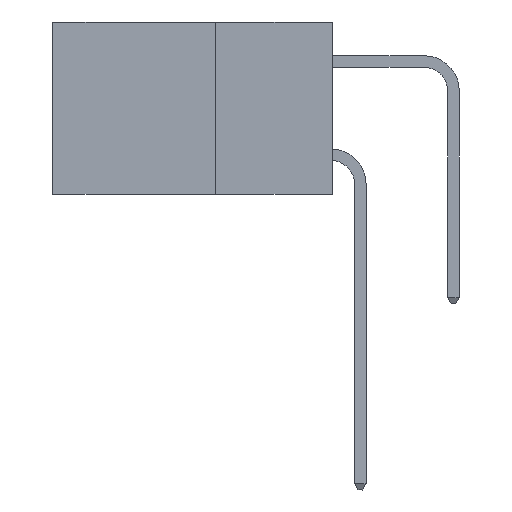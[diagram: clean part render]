
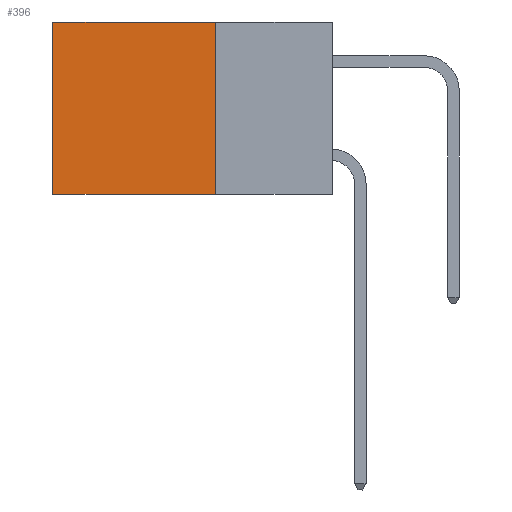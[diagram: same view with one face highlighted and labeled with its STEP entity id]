
A CAD part, left-side view. The second image highlights one B-rep face of the part: STEP entity #396.
In plain terms, the highlighted planar face has unit normal (-1, 0, 0).
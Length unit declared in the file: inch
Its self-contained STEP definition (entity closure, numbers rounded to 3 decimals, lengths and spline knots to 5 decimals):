
#341 = VECTOR ( 'NONE', #6211, 39.37008 ) ;
#396 = ADVANCED_FACE ( 'NONE', ( #12912 ), #11045, .F. ) ;
#566 = CARTESIAN_POINT ( 'NONE',  ( 0.298, 0.25, -0.37 ) ) ;
#772 = CARTESIAN_POINT ( 'NONE',  ( 0.298, 0.25, 0. ) ) ;
#829 = CARTESIAN_POINT ( 'NONE',  ( 0.298, 0.6, 0. ) ) ;
#966 = VERTEX_POINT ( 'NONE', #7988 ) ;
#1000 = VERTEX_POINT ( 'NONE', #829 ) ;
#1346 = VECTOR ( 'NONE', #3923, 39.37008 ) ;
#3240 = LINE ( 'NONE', #772, #341 ) ;
#3419 = EDGE_CURVE ( 'NONE', #1000, #5969, #4022, .T. ) ;
#3547 = DIRECTION ( 'NONE',  ( 0., 0., -1. ) ) ;
#3620 = CARTESIAN_POINT ( 'NONE',  ( 0.298, 0.25, -0.37 ) ) ;
#3923 = DIRECTION ( 'NONE',  ( 0., 1., 0. ) ) ;
#4022 = LINE ( 'NONE', #5436, #4364 ) ;
#4034 = EDGE_LOOP ( 'NONE', ( #12975, #11419, #5934, #10228 ) ) ;
#4364 = VECTOR ( 'NONE', #7153, 39.37008 ) ;
#4723 = DIRECTION ( 'NONE',  ( 0., 1., 0. ) ) ;
#5141 = DIRECTION ( 'NONE',  ( 1., 0., 0. ) ) ;
#5436 = CARTESIAN_POINT ( 'NONE',  ( 0.298, 0.6, 0. ) ) ;
#5738 = CARTESIAN_POINT ( 'NONE',  ( 0.298, 0.6, -0.37 ) ) ;
#5934 = ORIENTED_EDGE ( 'NONE', *, *, #12367, .F. ) ;
#5969 = VERTEX_POINT ( 'NONE', #5738 ) ;
#6114 = CARTESIAN_POINT ( 'NONE',  ( 0.298, 0.25, 0. ) ) ;
#6211 = DIRECTION ( 'NONE',  ( 0., 0., -1. ) ) ;
#6814 = LINE ( 'NONE', #6114, #1346 ) ;
#7153 = DIRECTION ( 'NONE',  ( 0., 0., -1. ) ) ;
#7988 = CARTESIAN_POINT ( 'NONE',  ( 0.298, 0.25, 0. ) ) ;
#8065 = CARTESIAN_POINT ( 'NONE',  ( 0.298, 0.25, 0. ) ) ;
#8953 = AXIS2_PLACEMENT_3D ( 'NONE', #8065, #5141, #3547 ) ;
#9716 = VECTOR ( 'NONE', #4723, 39.37008 ) ;
#10228 = ORIENTED_EDGE ( 'NONE', *, *, #12962, .T. ) ;
#11045 = PLANE ( 'NONE',  #8953 ) ;
#11419 = ORIENTED_EDGE ( 'NONE', *, *, #12072, .F. ) ;
#12072 = EDGE_CURVE ( 'NONE', #13535, #5969, #12490, .T. ) ;
#12367 = EDGE_CURVE ( 'NONE', #966, #13535, #3240, .T. ) ;
#12490 = LINE ( 'NONE', #3620, #9716 ) ;
#12912 = FACE_OUTER_BOUND ( 'NONE', #4034, .T. ) ;
#12962 = EDGE_CURVE ( 'NONE', #966, #1000, #6814, .T. ) ;
#12975 = ORIENTED_EDGE ( 'NONE', *, *, #3419, .T. ) ;
#13535 = VERTEX_POINT ( 'NONE', #566 ) ;
